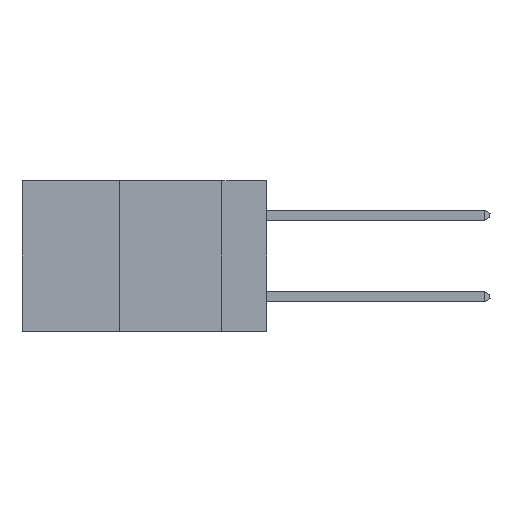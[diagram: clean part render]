
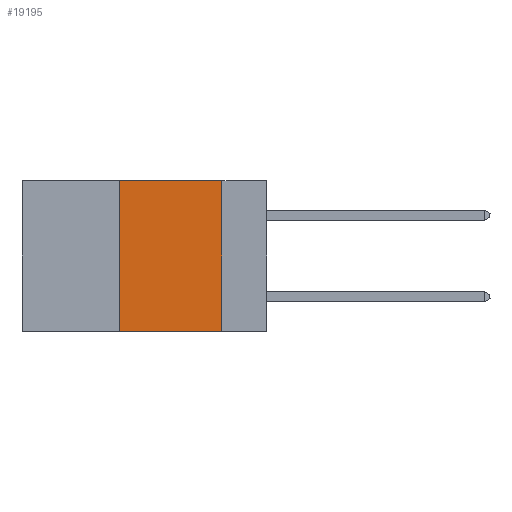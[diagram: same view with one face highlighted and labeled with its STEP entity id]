
A CAD part, left-side view. The second image highlights one B-rep face of the part: STEP entity #19195.
In plain terms, the highlighted planar face has unit normal (-1, 0, 0).
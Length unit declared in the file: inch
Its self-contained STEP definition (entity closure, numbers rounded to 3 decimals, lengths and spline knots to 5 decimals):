
#486 = CARTESIAN_POINT ( 'NONE',  ( 0., 0.6, 0. ) ) ;
#2073 = VERTEX_POINT ( 'NONE', #23778 ) ;
#2257 = CARTESIAN_POINT ( 'NONE',  ( 0., 0.36, 0. ) ) ;
#2532 = LINE ( 'NONE', #21380, #20505 ) ;
#5086 = DIRECTION ( 'NONE',  ( 1., 0., 0. ) ) ;
#6395 = VECTOR ( 'NONE', #11633, 39.37008 ) ;
#7622 = EDGE_LOOP ( 'NONE', ( #22453, #17131, #12247, #11636 ) ) ;
#7815 = EDGE_CURVE ( 'NONE', #9485, #2073, #15415, .T. ) ;
#8002 = EDGE_CURVE ( 'NONE', #13878, #2073, #2532, .T. ) ;
#9485 = VERTEX_POINT ( 'NONE', #12996 ) ;
#10249 = AXIS2_PLACEMENT_3D ( 'NONE', #16234, #5086, #18067 ) ;
#11633 = DIRECTION ( 'NONE',  ( 0., 0., 1. ) ) ;
#11636 = ORIENTED_EDGE ( 'NONE', *, *, #8002, .T. ) ;
#12247 = ORIENTED_EDGE ( 'NONE', *, *, #20262, .F. ) ;
#12329 = DIRECTION ( 'NONE',  ( 0., -1., 0. ) ) ;
#12996 = CARTESIAN_POINT ( 'NONE',  ( 0., 0.11, 0. ) ) ;
#13649 = DIRECTION ( 'NONE',  ( 0., -1., 0. ) ) ;
#13878 = VERTEX_POINT ( 'NONE', #18387 ) ;
#14257 = LINE ( 'NONE', #486, #23816 ) ;
#15415 = LINE ( 'NONE', #17299, #16572 ) ;
#15997 = CARTESIAN_POINT ( 'NONE',  ( 0., 0.36, 0. ) ) ;
#16234 = CARTESIAN_POINT ( 'NONE',  ( 0., 0.6, 0. ) ) ;
#16572 = VECTOR ( 'NONE', #20929, 39.37008 ) ;
#17131 = ORIENTED_EDGE ( 'NONE', *, *, #20969, .F. ) ;
#17246 = VERTEX_POINT ( 'NONE', #15997 ) ;
#17299 = CARTESIAN_POINT ( 'NONE',  ( 0., 0.11, 0. ) ) ;
#18067 = DIRECTION ( 'NONE',  ( 0., 0., -1. ) ) ;
#18387 = CARTESIAN_POINT ( 'NONE',  ( 0., 0.36, -0.37 ) ) ;
#19195 = ADVANCED_FACE ( 'NONE', ( #20293 ), #23384, .F. ) ;
#19963 = LINE ( 'NONE', #2257, #6395 ) ;
#20262 = EDGE_CURVE ( 'NONE', #13878, #17246, #19963, .T. ) ;
#20293 = FACE_OUTER_BOUND ( 'NONE', #7622, .T. ) ;
#20505 = VECTOR ( 'NONE', #12329, 39.37008 ) ;
#20929 = DIRECTION ( 'NONE',  ( 0., 0., -1. ) ) ;
#20969 = EDGE_CURVE ( 'NONE', #17246, #9485, #14257, .T. ) ;
#21380 = CARTESIAN_POINT ( 'NONE',  ( 0., 0.6, -0.37 ) ) ;
#22453 = ORIENTED_EDGE ( 'NONE', *, *, #7815, .F. ) ;
#23384 = PLANE ( 'NONE',  #10249 ) ;
#23778 = CARTESIAN_POINT ( 'NONE',  ( 0., 0.11, -0.37 ) ) ;
#23816 = VECTOR ( 'NONE', #13649, 39.37008 ) ;
